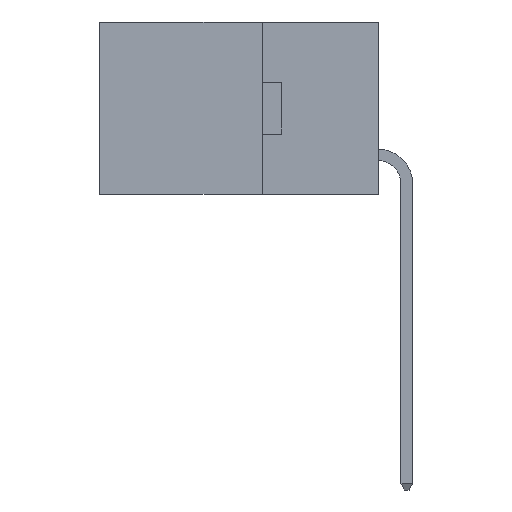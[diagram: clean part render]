
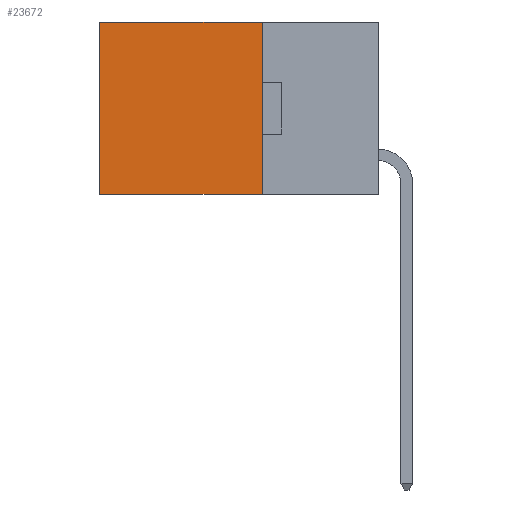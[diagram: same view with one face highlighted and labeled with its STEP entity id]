
A CAD part, left-side view. The second image highlights one B-rep face of the part: STEP entity #23672.
In plain terms, the highlighted planar face has unit normal (-1, 0, 0).
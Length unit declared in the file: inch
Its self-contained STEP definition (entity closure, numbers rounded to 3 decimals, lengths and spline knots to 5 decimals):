
#91 = ORIENTED_EDGE ( 'NONE', *, *, #5144, .T. ) ;
#247 = PLANE ( 'NONE',  #6462 ) ;
#863 = ORIENTED_EDGE ( 'NONE', *, *, #21920, .F. ) ;
#1808 = VERTEX_POINT ( 'NONE', #13836 ) ;
#2328 = DIRECTION ( 'NONE',  ( 1., 0., 0. ) ) ;
#2600 = CARTESIAN_POINT ( 'NONE',  ( 0.2615, 0.6, -0.37 ) ) ;
#4818 = EDGE_CURVE ( 'NONE', #6269, #21879, #23288, .T. ) ;
#4906 = DIRECTION ( 'NONE',  ( 0., 1., 0. ) ) ;
#5144 = EDGE_CURVE ( 'NONE', #15584, #6269, #13679, .T. ) ;
#5356 = VECTOR ( 'NONE', #4906, 39.37008 ) ;
#6154 = DIRECTION ( 'NONE',  ( 0., 0., -1. ) ) ;
#6269 = VERTEX_POINT ( 'NONE', #7096 ) ;
#6344 = VECTOR ( 'NONE', #6154, 39.37008 ) ;
#6356 = CARTESIAN_POINT ( 'NONE',  ( 0.2615, 0.25, -0.37 ) ) ;
#6462 = AXIS2_PLACEMENT_3D ( 'NONE', #6356, #2328, #16604 ) ;
#6504 = VECTOR ( 'NONE', #19678, 39.37008 ) ;
#7096 = CARTESIAN_POINT ( 'NONE',  ( 0.2615, 0.6, 0. ) ) ;
#8202 = CARTESIAN_POINT ( 'NONE',  ( 0.2615, 0.6, -0.37 ) ) ;
#8250 = VECTOR ( 'NONE', #13469, 39.37008 ) ;
#10186 = LINE ( 'NONE', #17138, #5356 ) ;
#11483 = CARTESIAN_POINT ( 'NONE',  ( 0.2615, 0.25, -0.37 ) ) ;
#11949 = LINE ( 'NONE', #11483, #6504 ) ;
#13469 = DIRECTION ( 'NONE',  ( 0., 1., 0. ) ) ;
#13679 = LINE ( 'NONE', #15404, #8250 ) ;
#13836 = CARTESIAN_POINT ( 'NONE',  ( 0.2615, 0.25, -0.37 ) ) ;
#15404 = CARTESIAN_POINT ( 'NONE',  ( 0.2615, 0.25, 0. ) ) ;
#15584 = VERTEX_POINT ( 'NONE', #21381 ) ;
#15997 = ORIENTED_EDGE ( 'NONE', *, *, #4818, .T. ) ;
#16604 = DIRECTION ( 'NONE',  ( 0., 0., -1. ) ) ;
#17138 = CARTESIAN_POINT ( 'NONE',  ( 0.2615, 0.25, -0.37 ) ) ;
#19338 = EDGE_LOOP ( 'NONE', ( #15997, #863, #25231, #91 ) ) ;
#19678 = DIRECTION ( 'NONE',  ( 0., 0., -1. ) ) ;
#21381 = CARTESIAN_POINT ( 'NONE',  ( 0.2615, 0.25, 0. ) ) ;
#21879 = VERTEX_POINT ( 'NONE', #2600 ) ;
#21920 = EDGE_CURVE ( 'NONE', #1808, #21879, #10186, .T. ) ;
#23288 = LINE ( 'NONE', #8202, #6344 ) ;
#23672 = ADVANCED_FACE ( 'NONE', ( #24462 ), #247, .F. ) ;
#24462 = FACE_OUTER_BOUND ( 'NONE', #19338, .T. ) ;
#25112 = EDGE_CURVE ( 'NONE', #15584, #1808, #11949, .T. ) ;
#25231 = ORIENTED_EDGE ( 'NONE', *, *, #25112, .F. ) ;
